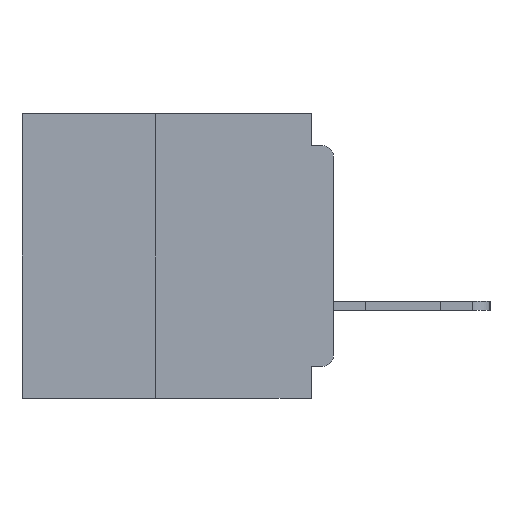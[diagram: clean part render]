
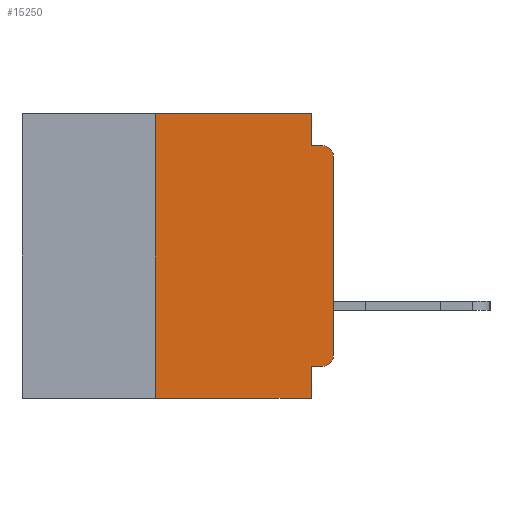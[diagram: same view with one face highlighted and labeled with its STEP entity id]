
A CAD part, left-side view. The second image highlights one B-rep face of the part: STEP entity #15250.
In plain terms, the highlighted planar face has unit normal (-1, 0, 0).
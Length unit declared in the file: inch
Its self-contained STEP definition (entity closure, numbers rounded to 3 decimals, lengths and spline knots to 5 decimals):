
#489 = EDGE_CURVE ( 'NONE', #2180, #4799, #44991, .T. ) ;
#1760 = AXIS2_PLACEMENT_3D ( 'NONE', #23357, #2195, #26903 ) ;
#1934 = CARTESIAN_POINT ( 'NONE',  ( 0., 0.031, -0.355 ) ) ;
#2180 = VERTEX_POINT ( 'NONE', #34843 ) ;
#2195 = DIRECTION ( 'NONE',  ( -1., 0., 0. ) ) ;
#2384 = LINE ( 'NONE', #26153, #10691 ) ;
#2739 = ORIENTED_EDGE ( 'NONE', *, *, #8888, .T. ) ;
#4169 = CARTESIAN_POINT ( 'NONE',  ( 0., 0.25, -0.4 ) ) ;
#4547 = FACE_OUTER_BOUND ( 'NONE', #15188, .T. ) ;
#4695 = DIRECTION ( 'NONE',  ( 0., 1., 0. ) ) ;
#4799 = VERTEX_POINT ( 'NONE', #32294 ) ;
#5599 = LINE ( 'NONE', #32325, #42038 ) ;
#6396 = CARTESIAN_POINT ( 'NONE',  ( 0., 0.015, -0.34 ) ) ;
#6406 = ORIENTED_EDGE ( 'NONE', *, *, #10921, .T. ) ;
#6690 = CARTESIAN_POINT ( 'NONE',  ( 0., 0.25, -0.4 ) ) ;
#6790 = ORIENTED_EDGE ( 'NONE', *, *, #39927, .F. ) ;
#6863 = VERTEX_POINT ( 'NONE', #9594 ) ;
#8109 = CIRCLE ( 'NONE', #38763, 0.015 ) ;
#8537 = DIRECTION ( 'NONE',  ( 0., -1., 0. ) ) ;
#8888 = EDGE_CURVE ( 'NONE', #9042, #6863, #5599, .T. ) ;
#9002 = DIRECTION ( 'NONE',  ( 0., -1., 0. ) ) ;
#9042 = VERTEX_POINT ( 'NONE', #43690 ) ;
#9473 = PLANE ( 'NONE',  #9888 ) ;
#9594 = CARTESIAN_POINT ( 'NONE',  ( 0., 0., -0.06 ) ) ;
#9888 = AXIS2_PLACEMENT_3D ( 'NONE', #34167, #37721, #16593 ) ;
#9989 = DIRECTION ( 'NONE',  ( 0., 0., -1. ) ) ;
#10037 = CARTESIAN_POINT ( 'NONE',  ( 0., 0.437, 0. ) ) ;
#10196 = LINE ( 'NONE', #43435, #17369 ) ;
#10280 = VECTOR ( 'NONE', #41044, 39.37008 ) ;
#10691 = VECTOR ( 'NONE', #8537, 39.37008 ) ;
#10785 = ORIENTED_EDGE ( 'NONE', *, *, #38009, .F. ) ;
#10921 = EDGE_CURVE ( 'NONE', #6863, #18718, #21456, .T. ) ;
#12274 = VERTEX_POINT ( 'NONE', #6690 ) ;
#12496 = LINE ( 'NONE', #37373, #10280 ) ;
#12762 = CARTESIAN_POINT ( 'NONE',  ( 0., 0.031, -0.4 ) ) ;
#12841 = ORIENTED_EDGE ( 'NONE', *, *, #32790, .T. ) ;
#15188 = EDGE_LOOP ( 'NONE', ( #2739, #6406, #34690, #25192, #33974, #10785, #12841, #6790, #24247, #39535 ) ) ;
#15250 = ADVANCED_FACE ( 'NONE', ( #4547 ), #9473, .F. ) ;
#16593 = DIRECTION ( 'NONE',  ( 0., 0., -1. ) ) ;
#16876 = CARTESIAN_POINT ( 'NONE',  ( 0., 0.015, -0.355 ) ) ;
#17369 = VECTOR ( 'NONE', #4695, 39.37008 ) ;
#17799 = DIRECTION ( 'NONE',  ( 0., 0., -1. ) ) ;
#18181 = VERTEX_POINT ( 'NONE', #1934 ) ;
#18718 = VERTEX_POINT ( 'NONE', #22451 ) ;
#19307 = VECTOR ( 'NONE', #39513, 39.37008 ) ;
#19907 = EDGE_CURVE ( 'NONE', #4799, #31495, #29015, .T. ) ;
#21456 = CIRCLE ( 'NONE', #1760, 0.015 ) ;
#22451 = CARTESIAN_POINT ( 'NONE',  ( 0., 0.015, -0.045 ) ) ;
#22979 = VECTOR ( 'NONE', #35126, 39.37008 ) ;
#23357 = CARTESIAN_POINT ( 'NONE',  ( 0., 0.015, -0.06 ) ) ;
#24247 = ORIENTED_EDGE ( 'NONE', *, *, #33828, .F. ) ;
#25192 = ORIENTED_EDGE ( 'NONE', *, *, #19907, .F. ) ;
#26153 = CARTESIAN_POINT ( 'NONE',  ( 0., 0., -0.045 ) ) ;
#26903 = DIRECTION ( 'NONE',  ( 0., 0., -1. ) ) ;
#27931 = EDGE_CURVE ( 'NONE', #34575, #9042, #8109, .T. ) ;
#29015 = LINE ( 'NONE', #42447, #37321 ) ;
#31110 = DIRECTION ( 'NONE',  ( -1., 0., 0. ) ) ;
#31495 = VERTEX_POINT ( 'NONE', #42151 ) ;
#31568 = CARTESIAN_POINT ( 'NONE',  ( 0., 0.437, -0.4 ) ) ;
#32294 = CARTESIAN_POINT ( 'NONE',  ( 0., 0.031, 0. ) ) ;
#32325 = CARTESIAN_POINT ( 'NONE',  ( 0., 0., 0. ) ) ;
#32790 = EDGE_CURVE ( 'NONE', #12274, #33978, #41719, .T. ) ;
#33828 = EDGE_CURVE ( 'NONE', #34575, #18181, #10196, .T. ) ;
#33974 = ORIENTED_EDGE ( 'NONE', *, *, #489, .F. ) ;
#33978 = VERTEX_POINT ( 'NONE', #12762 ) ;
#34167 = CARTESIAN_POINT ( 'NONE',  ( 0., 0.437, 0. ) ) ;
#34356 = EDGE_CURVE ( 'NONE', #31495, #18718, #2384, .T. ) ;
#34575 = VERTEX_POINT ( 'NONE', #16876 ) ;
#34690 = ORIENTED_EDGE ( 'NONE', *, *, #34356, .F. ) ;
#34843 = CARTESIAN_POINT ( 'NONE',  ( 0., 0.25, 0. ) ) ;
#35126 = DIRECTION ( 'NONE',  ( 0., -1., 0. ) ) ;
#35682 = VECTOR ( 'NONE', #9002, 39.37008 ) ;
#37321 = VECTOR ( 'NONE', #17799, 39.37008 ) ;
#37373 = CARTESIAN_POINT ( 'NONE',  ( 0., 0.031, -0.4 ) ) ;
#37721 = DIRECTION ( 'NONE',  ( 1., 0., 0. ) ) ;
#38009 = EDGE_CURVE ( 'NONE', #12274, #2180, #39167, .T. ) ;
#38763 = AXIS2_PLACEMENT_3D ( 'NONE', #6396, #31110, #9989 ) ;
#39167 = LINE ( 'NONE', #4169, #19307 ) ;
#39413 = DIRECTION ( 'NONE',  ( 0., 0., 1. ) ) ;
#39513 = DIRECTION ( 'NONE',  ( 0., 0., 1. ) ) ;
#39535 = ORIENTED_EDGE ( 'NONE', *, *, #27931, .T. ) ;
#39927 = EDGE_CURVE ( 'NONE', #18181, #33978, #12496, .T. ) ;
#41044 = DIRECTION ( 'NONE',  ( 0., 0., -1. ) ) ;
#41719 = LINE ( 'NONE', #31568, #22979 ) ;
#42038 = VECTOR ( 'NONE', #39413, 39.37008 ) ;
#42151 = CARTESIAN_POINT ( 'NONE',  ( 0., 0.031, -0.045 ) ) ;
#42447 = CARTESIAN_POINT ( 'NONE',  ( 0., 0.031, 0. ) ) ;
#43435 = CARTESIAN_POINT ( 'NONE',  ( 0., 0., -0.355 ) ) ;
#43690 = CARTESIAN_POINT ( 'NONE',  ( 0., 0., -0.34 ) ) ;
#44991 = LINE ( 'NONE', #10037, #35682 ) ;
